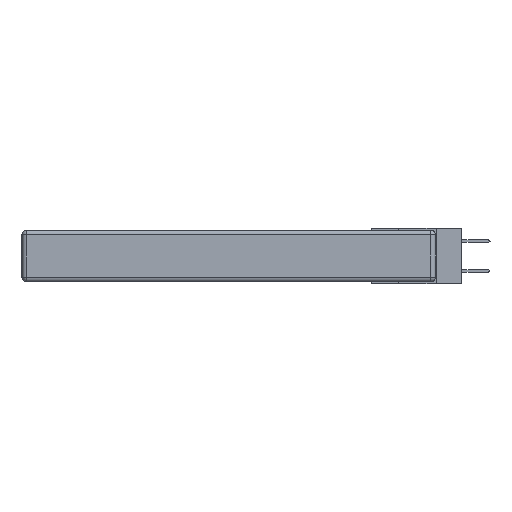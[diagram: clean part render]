
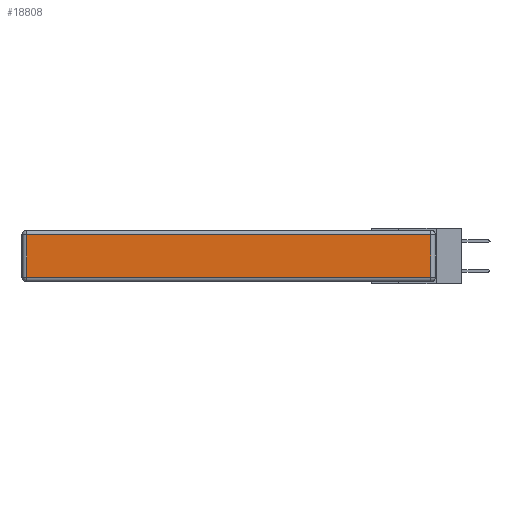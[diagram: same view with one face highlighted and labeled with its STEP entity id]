
A CAD part, left-side view. The second image highlights one B-rep face of the part: STEP entity #18808.
In plain terms, the highlighted planar face has unit normal (-1, 0, 0).
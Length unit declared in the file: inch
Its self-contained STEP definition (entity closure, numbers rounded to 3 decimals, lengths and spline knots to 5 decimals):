
#1733 = CARTESIAN_POINT ( 'NONE',  ( 0., 0.03, -0.343 ) ) ;
#2156 = VECTOR ( 'NONE', #20307, 39.37008 ) ;
#2569 = LINE ( 'NONE', #6723, #8957 ) ;
#2757 = EDGE_CURVE ( 'NONE', #15356, #5523, #26300, .T. ) ;
#4111 = LINE ( 'NONE', #6481, #7289 ) ;
#4490 = DIRECTION ( 'NONE',  ( 0., 1., 0. ) ) ;
#4604 = CARTESIAN_POINT ( 'NONE',  ( 0., 2.72, -0.313 ) ) ;
#5523 = VERTEX_POINT ( 'NONE', #4604 ) ;
#6481 = CARTESIAN_POINT ( 'NONE',  ( 0., 0., -0.313 ) ) ;
#6723 = CARTESIAN_POINT ( 'NONE',  ( 0., 2.75, -0.03 ) ) ;
#7289 = VECTOR ( 'NONE', #15304, 39.37008 ) ;
#8433 = ORIENTED_EDGE ( 'NONE', *, *, #17567, .T. ) ;
#8957 = VECTOR ( 'NONE', #4490, 39.37008 ) ;
#9208 = EDGE_CURVE ( 'NONE', #5523, #24971, #4111, .T. ) ;
#9894 = ORIENTED_EDGE ( 'NONE', *, *, #2757, .T. ) ;
#9922 = DIRECTION ( 'NONE',  ( 0., 0., 1. ) ) ;
#11841 = DIRECTION ( 'NONE',  ( -1., 0., 0. ) ) ;
#12157 = CARTESIAN_POINT ( 'NONE',  ( 0., 0.03, -0.03 ) ) ;
#12481 = EDGE_LOOP ( 'NONE', ( #22712, #13593, #8433, #9894 ) ) ;
#13593 = ORIENTED_EDGE ( 'NONE', *, *, #18867, .T. ) ;
#14081 = CARTESIAN_POINT ( 'NONE',  ( 0., 0., -0.343 ) ) ;
#15077 = CARTESIAN_POINT ( 'NONE',  ( 0., 2.72, -0.343 ) ) ;
#15304 = DIRECTION ( 'NONE',  ( 0., -1., 0. ) ) ;
#15356 = VERTEX_POINT ( 'NONE', #15836 ) ;
#15836 = CARTESIAN_POINT ( 'NONE',  ( 0., 2.72, -0.03 ) ) ;
#15847 = PLANE ( 'NONE',  #20677 ) ;
#17567 = EDGE_CURVE ( 'NONE', #21620, #15356, #2569, .T. ) ;
#18808 = ADVANCED_FACE ( 'NONE', ( #23959 ), #15847, .T. ) ;
#18867 = EDGE_CURVE ( 'NONE', #24971, #21620, #19456, .T. ) ;
#19456 = LINE ( 'NONE', #1733, #2156 ) ;
#20307 = DIRECTION ( 'NONE',  ( 0., 0., 1. ) ) ;
#20677 = AXIS2_PLACEMENT_3D ( 'NONE', #14081, #11841, #9922 ) ;
#21620 = VERTEX_POINT ( 'NONE', #12157 ) ;
#22712 = ORIENTED_EDGE ( 'NONE', *, *, #9208, .T. ) ;
#23272 = DIRECTION ( 'NONE',  ( 0., 0., -1. ) ) ;
#23959 = FACE_OUTER_BOUND ( 'NONE', #12481, .T. ) ;
#24971 = VERTEX_POINT ( 'NONE', #25162 ) ;
#25013 = VECTOR ( 'NONE', #23272, 39.37008 ) ;
#25162 = CARTESIAN_POINT ( 'NONE',  ( 0., 0.03, -0.313 ) ) ;
#26300 = LINE ( 'NONE', #15077, #25013 ) ;
